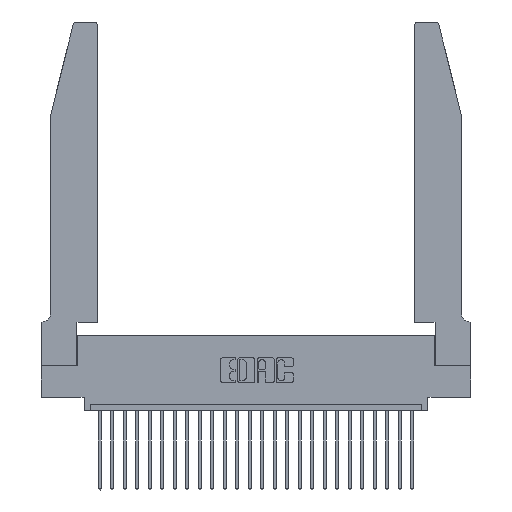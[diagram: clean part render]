
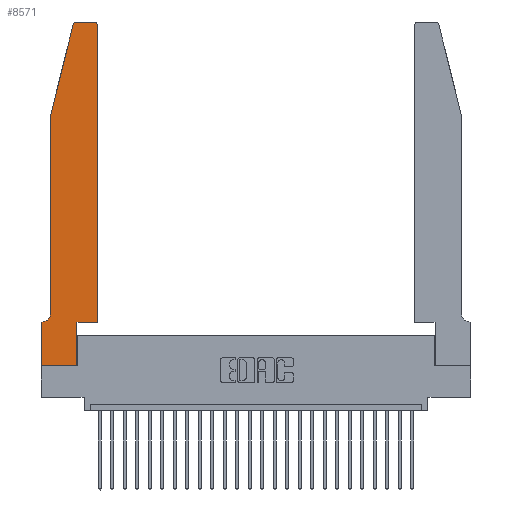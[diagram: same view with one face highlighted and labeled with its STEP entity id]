
A CAD part, top view. The second image highlights one B-rep face of the part: STEP entity #8571.
In plain terms, the highlighted planar face has unit normal (0, 0, 1).
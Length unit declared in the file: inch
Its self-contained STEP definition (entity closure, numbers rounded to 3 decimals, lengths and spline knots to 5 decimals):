
#109 = CARTESIAN_POINT ( 'NONE',  ( 0.2865, 0.35, 0.37 ) ) ;
#147 = CARTESIAN_POINT ( 'NONE',  ( 0., 0., 0.37 ) ) ;
#244 = VERTEX_POINT ( 'NONE', #5878 ) ;
#288 = VECTOR ( 'NONE', #22670, 39.37008 ) ;
#314 = LINE ( 'NONE', #15790, #979 ) ;
#366 = CARTESIAN_POINT ( 'NONE',  ( 0.4505, 0.35, 0.37 ) ) ;
#865 = CARTESIAN_POINT ( 'NONE',  ( 0.4505, 0.35, 0.37 ) ) ;
#979 = VECTOR ( 'NONE', #21615, 39.37008 ) ;
#1289 = EDGE_CURVE ( 'NONE', #17883, #10375, #6751, .T. ) ;
#1307 = VERTEX_POINT ( 'NONE', #9485 ) ;
#1509 = LINE ( 'NONE', #865, #2172 ) ;
#1631 = FACE_OUTER_BOUND ( 'NONE', #18538, .T. ) ;
#1790 = VECTOR ( 'NONE', #9505, 39.37008 ) ;
#1953 = DIRECTION ( 'NONE',  ( 1., 0., 0. ) ) ;
#1995 = EDGE_CURVE ( 'NONE', #21364, #7119, #14133, .T. ) ;
#2018 = CARTESIAN_POINT ( 'NONE',  ( 0.0755, 2., 0.37 ) ) ;
#2172 = VECTOR ( 'NONE', #23510, 39.37008 ) ;
#2742 = VECTOR ( 'NONE', #7765, 39.37008 ) ;
#3044 = ORIENTED_EDGE ( 'NONE', *, *, #22659, .T. ) ;
#3247 = EDGE_CURVE ( 'NONE', #20091, #21364, #1509, .T. ) ;
#3689 = EDGE_CURVE ( 'NONE', #1307, #10471, #19815, .T. ) ;
#3736 = DIRECTION ( 'NONE',  ( 0., 0., 1. ) ) ;
#4185 = LINE ( 'NONE', #12259, #288 ) ;
#4248 = VERTEX_POINT ( 'NONE', #16768 ) ;
#4332 = LINE ( 'NONE', #2018, #7518 ) ;
#4396 = CARTESIAN_POINT ( 'NONE',  ( 0.0055, 0.42, 0.37 ) ) ;
#4660 = EDGE_CURVE ( 'NONE', #4248, #1307, #4332, .T. ) ;
#4706 = ORIENTED_EDGE ( 'NONE', *, *, #1289, .T. ) ;
#5647 = CARTESIAN_POINT ( 'NONE',  ( 0.2605, 2.75, 0.37 ) ) ;
#5878 = CARTESIAN_POINT ( 'NONE',  ( 0.2865, 0., 0.37 ) ) ;
#6751 = LINE ( 'NONE', #147, #15136 ) ;
#7027 = ORIENTED_EDGE ( 'NONE', *, *, #3689, .T. ) ;
#7119 = VERTEX_POINT ( 'NONE', #20589 ) ;
#7518 = VECTOR ( 'NONE', #16403, 39.37008 ) ;
#7765 = DIRECTION ( 'NONE',  ( -1., 0., 0. ) ) ;
#8184 = LINE ( 'NONE', #5647, #2742 ) ;
#8222 = VECTOR ( 'NONE', #14927, 39.37008 ) ;
#8345 = DIRECTION ( 'NONE',  ( 1., 0., 0. ) ) ;
#8417 = DIRECTION ( 'NONE',  ( -1., 0., 0. ) ) ;
#8571 = ADVANCED_FACE ( 'NONE', ( #1631 ), #20181, .T. ) ;
#9086 = DIRECTION ( 'NONE',  ( 0., 1., 0. ) ) ;
#9427 = CARTESIAN_POINT ( 'NONE',  ( 0., 0., 0.37 ) ) ;
#9485 = CARTESIAN_POINT ( 'NONE',  ( 0.0755, 2., 0.37 ) ) ;
#9505 = DIRECTION ( 'NONE',  ( 1., 0., 0. ) ) ;
#10375 = VERTEX_POINT ( 'NONE', #20706 ) ;
#10471 = VERTEX_POINT ( 'NONE', #12873 ) ;
#10903 = VECTOR ( 'NONE', #9086, 39.37008 ) ;
#11007 = ORIENTED_EDGE ( 'NONE', *, *, #3247, .T. ) ;
#11016 = AXIS2_PLACEMENT_3D ( 'NONE', #26346, #11902, #14089 ) ;
#11197 = EDGE_CURVE ( 'NONE', #10375, #244, #21073, .T. ) ;
#11902 = DIRECTION ( 'NONE',  ( 0., 0., 1. ) ) ;
#11963 = EDGE_CURVE ( 'NONE', #23928, #4248, #25833, .T. ) ;
#12179 = CARTESIAN_POINT ( 'NONE',  ( 0., 0.35, 0.37 ) ) ;
#12259 = CARTESIAN_POINT ( 'NONE',  ( 0.2865, 0.35, 0.37 ) ) ;
#12266 = ORIENTED_EDGE ( 'NONE', *, *, #15611, .T. ) ;
#12873 = CARTESIAN_POINT ( 'NONE',  ( 0.0755, 0.42, 0.37 ) ) ;
#13056 = ORIENTED_EDGE ( 'NONE', *, *, #4660, .T. ) ;
#14089 = DIRECTION ( 'NONE',  ( 1., 0., 0. ) ) ;
#14133 = LINE ( 'NONE', #25672, #10903 ) ;
#14356 = VERTEX_POINT ( 'NONE', #23260 ) ;
#14702 = ORIENTED_EDGE ( 'NONE', *, *, #11963, .T. ) ;
#14927 = DIRECTION ( 'NONE',  ( 0., -1., 0. ) ) ;
#15136 = VECTOR ( 'NONE', #26564, 39.37008 ) ;
#15611 = EDGE_CURVE ( 'NONE', #10471, #17784, #21480, .T. ) ;
#15790 = CARTESIAN_POINT ( 'NONE',  ( 0.0755, 0.35, 0.37 ) ) ;
#16282 = EDGE_CURVE ( 'NONE', #7119, #14356, #25572, .T. ) ;
#16403 = DIRECTION ( 'NONE',  ( -0.239, -0.971, 0. ) ) ;
#16488 = CARTESIAN_POINT ( 'NONE',  ( 0.4205, 2.72, 0.37 ) ) ;
#16768 = CARTESIAN_POINT ( 'NONE',  ( 0.25487, 2.72718, 0.37 ) ) ;
#16837 = DIRECTION ( 'NONE',  ( 0., 0., 1. ) ) ;
#17784 = VERTEX_POINT ( 'NONE', #20042 ) ;
#17883 = VERTEX_POINT ( 'NONE', #18419 ) ;
#18419 = CARTESIAN_POINT ( 'NONE',  ( 0., 0.35, 0.37 ) ) ;
#18538 = EDGE_LOOP ( 'NONE', ( #19802, #14702, #13056, #7027, #12266, #3044, #4706, #20588, #19803, #11007, #22483, #20617 ) ) ;
#19802 = ORIENTED_EDGE ( 'NONE', *, *, #20551, .T. ) ;
#19803 = ORIENTED_EDGE ( 'NONE', *, *, #23008, .T. ) ;
#19815 = LINE ( 'NONE', #25195, #8222 ) ;
#20042 = CARTESIAN_POINT ( 'NONE',  ( 0.0055, 0.35, 0.37 ) ) ;
#20091 = VERTEX_POINT ( 'NONE', #109 ) ;
#20181 = PLANE ( 'NONE',  #23537 ) ;
#20551 = EDGE_CURVE ( 'NONE', #14356, #23928, #8184, .T. ) ;
#20588 = ORIENTED_EDGE ( 'NONE', *, *, #11197, .T. ) ;
#20589 = CARTESIAN_POINT ( 'NONE',  ( 0.4505, 2.72, 0.37 ) ) ;
#20617 = ORIENTED_EDGE ( 'NONE', *, *, #16282, .T. ) ;
#20706 = CARTESIAN_POINT ( 'NONE',  ( 0., 0., 0.37 ) ) ;
#21073 = LINE ( 'NONE', #9427, #1790 ) ;
#21364 = VERTEX_POINT ( 'NONE', #366 ) ;
#21480 = CIRCLE ( 'NONE', #21732, 0.07 ) ;
#21615 = DIRECTION ( 'NONE',  ( -1., 0., 0. ) ) ;
#21732 = AXIS2_PLACEMENT_3D ( 'NONE', #4396, #23143, #8417 ) ;
#22483 = ORIENTED_EDGE ( 'NONE', *, *, #1995, .T. ) ;
#22659 = EDGE_CURVE ( 'NONE', #17784, #17883, #314, .T. ) ;
#22670 = DIRECTION ( 'NONE',  ( 0., 1., 0. ) ) ;
#23008 = EDGE_CURVE ( 'NONE', #244, #20091, #4185, .T. ) ;
#23143 = DIRECTION ( 'NONE',  ( 0., 0., -1. ) ) ;
#23260 = CARTESIAN_POINT ( 'NONE',  ( 0.4205, 2.75, 0.37 ) ) ;
#23510 = DIRECTION ( 'NONE',  ( 1., 0., 0. ) ) ;
#23537 = AXIS2_PLACEMENT_3D ( 'NONE', #12179, #3736, #1953 ) ;
#23928 = VERTEX_POINT ( 'NONE', #25642 ) ;
#24979 = AXIS2_PLACEMENT_3D ( 'NONE', #16488, #16837, #8345 ) ;
#25195 = CARTESIAN_POINT ( 'NONE',  ( 0.0755, 2., 0.37 ) ) ;
#25572 = CIRCLE ( 'NONE', #24979, 0.03 ) ;
#25642 = CARTESIAN_POINT ( 'NONE',  ( 0.284, 2.75, 0.37 ) ) ;
#25672 = CARTESIAN_POINT ( 'NONE',  ( 0.4505, 0.35, 0.37 ) ) ;
#25833 = CIRCLE ( 'NONE', #11016, 0.03 ) ;
#26346 = CARTESIAN_POINT ( 'NONE',  ( 0.284, 2.72, 0.37 ) ) ;
#26564 = DIRECTION ( 'NONE',  ( 0., -1., 0. ) ) ;
